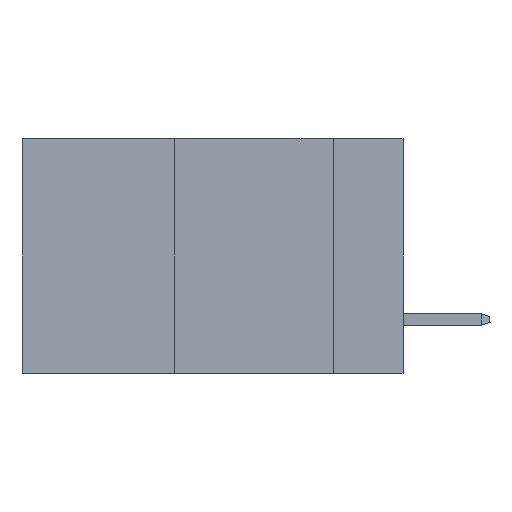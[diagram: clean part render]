
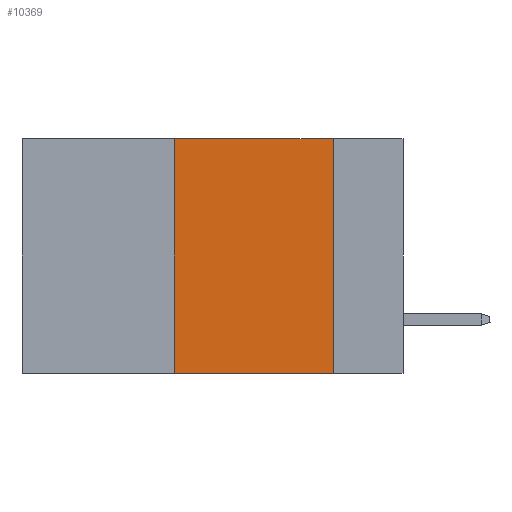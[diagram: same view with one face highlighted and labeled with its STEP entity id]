
A CAD part, left-side view. The second image highlights one B-rep face of the part: STEP entity #10369.
In plain terms, the highlighted planar face has unit normal (-1, 0, 0).
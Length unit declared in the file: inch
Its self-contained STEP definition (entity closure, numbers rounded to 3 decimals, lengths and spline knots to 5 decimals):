
#690 = CARTESIAN_POINT ( 'NONE',  ( 0., 0.6, 0. ) ) ;
#873 = DIRECTION ( 'NONE',  ( 1., 0., 0. ) ) ;
#957 = CARTESIAN_POINT ( 'NONE',  ( 0., 0.11, 0. ) ) ;
#1846 = VERTEX_POINT ( 'NONE', #16735 ) ;
#2377 = DIRECTION ( 'NONE',  ( 0., 0., -1. ) ) ;
#2565 = LINE ( 'NONE', #957, #14063 ) ;
#2591 = VECTOR ( 'NONE', #3770, 39.37008 ) ;
#3663 = EDGE_CURVE ( 'NONE', #14794, #1846, #2565, .T. ) ;
#3770 = DIRECTION ( 'NONE',  ( 0., -1., 0. ) ) ;
#3979 = CARTESIAN_POINT ( 'NONE',  ( 0., 0.6, 0. ) ) ;
#5766 = EDGE_CURVE ( 'NONE', #18758, #16041, #6950, .T. ) ;
#6679 = FACE_OUTER_BOUND ( 'NONE', #8275, .T. ) ;
#6950 = LINE ( 'NONE', #11427, #9818 ) ;
#6995 = CARTESIAN_POINT ( 'NONE',  ( 0., 0.11, 0. ) ) ;
#7352 = VECTOR ( 'NONE', #13815, 39.37008 ) ;
#8174 = CARTESIAN_POINT ( 'NONE',  ( 0., 0.36, 0. ) ) ;
#8275 = EDGE_LOOP ( 'NONE', ( #17884, #9697, #14921, #18820 ) ) ;
#9697 = ORIENTED_EDGE ( 'NONE', *, *, #12498, .F. ) ;
#9818 = VECTOR ( 'NONE', #11331, 39.37008 ) ;
#10369 = ADVANCED_FACE ( 'NONE', ( #6679 ), #15098, .F. ) ;
#10747 = LINE ( 'NONE', #15052, #2591 ) ;
#11331 = DIRECTION ( 'NONE',  ( 0., 0., 1. ) ) ;
#11427 = CARTESIAN_POINT ( 'NONE',  ( 0., 0.36, 0. ) ) ;
#12498 = EDGE_CURVE ( 'NONE', #16041, #14794, #16066, .T. ) ;
#13765 = CARTESIAN_POINT ( 'NONE',  ( 0., 0.36, -0.37 ) ) ;
#13815 = DIRECTION ( 'NONE',  ( 0., -1., 0. ) ) ;
#14063 = VECTOR ( 'NONE', #15557, 39.37008 ) ;
#14794 = VERTEX_POINT ( 'NONE', #6995 ) ;
#14921 = ORIENTED_EDGE ( 'NONE', *, *, #5766, .F. ) ;
#15052 = CARTESIAN_POINT ( 'NONE',  ( 0., 0.6, -0.37 ) ) ;
#15098 = PLANE ( 'NONE',  #17403 ) ;
#15557 = DIRECTION ( 'NONE',  ( 0., 0., -1. ) ) ;
#16041 = VERTEX_POINT ( 'NONE', #8174 ) ;
#16066 = LINE ( 'NONE', #3979, #7352 ) ;
#16735 = CARTESIAN_POINT ( 'NONE',  ( 0., 0.11, -0.37 ) ) ;
#17403 = AXIS2_PLACEMENT_3D ( 'NONE', #690, #873, #2377 ) ;
#17884 = ORIENTED_EDGE ( 'NONE', *, *, #3663, .F. ) ;
#18270 = EDGE_CURVE ( 'NONE', #18758, #1846, #10747, .T. ) ;
#18758 = VERTEX_POINT ( 'NONE', #13765 ) ;
#18820 = ORIENTED_EDGE ( 'NONE', *, *, #18270, .T. ) ;
